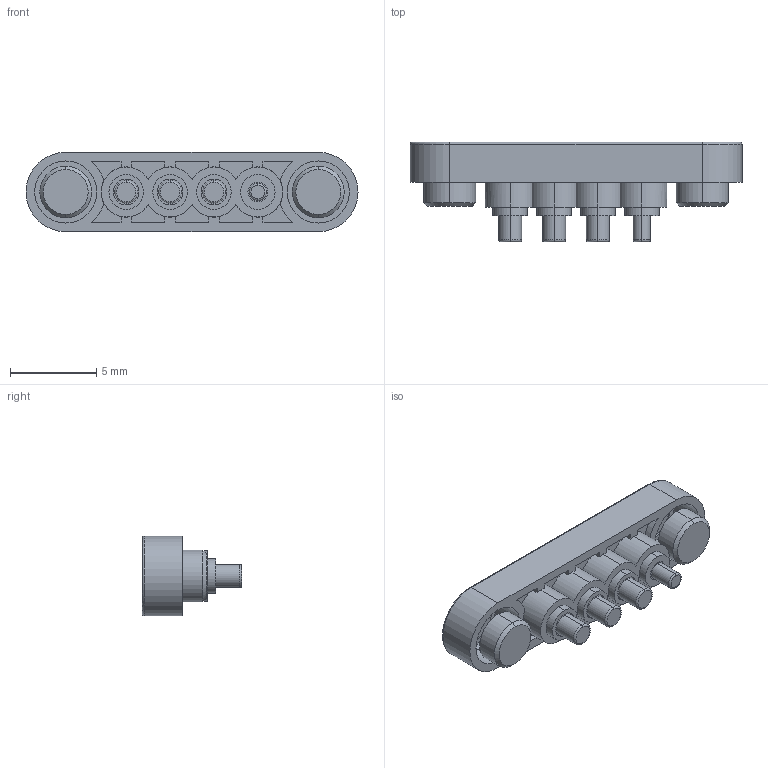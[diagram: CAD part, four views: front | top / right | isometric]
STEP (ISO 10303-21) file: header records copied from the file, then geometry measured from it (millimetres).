
FILE_DESCRIPTION (( 'STEP AP214' ), '1' );
FILE_NAME ('686E0422250110E.STEP', '2023-05-01T19:46:00', ( '' ), ( '' ), 'SwSTEP 2.0', 'SolidWorks 2020', '' );
FILE_SCHEMA (( 'AUTOMOTIVE_DESIGN' ));
Length unit declared in the file: inch
Products named in the file (1): 686E0422250110E
Bounding box: 19.22 x 5.75 x 4.6 mm (x, y, z)
Volume: 217.3 mm3; surface area: 484.7 mm2
Topology: 9 solids, 9 shells, 187 faces, 446 edges, 286 vertices
Faces by surface type: plane 73, cylinder 72, torus 16, bspline 14, cone 12
Entity records: 6708 total; most frequent: CARTESIAN_POINT 1742, DIRECTION 948, ORIENTED_EDGE 876, EDGE_CURVE 438, AXIS2_PLACEMENT_3D 364, VERTEX_POINT 286, VECTOR 220, LINE 220
